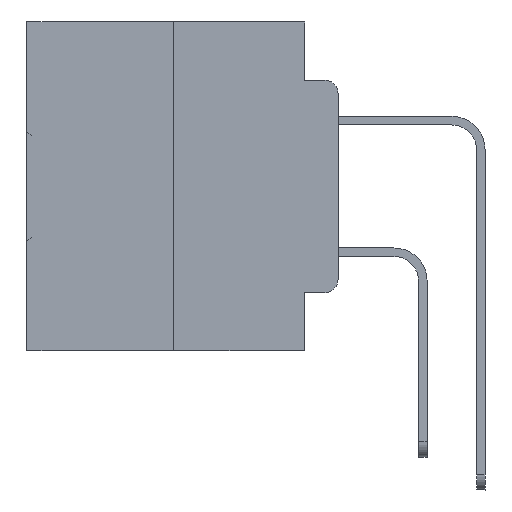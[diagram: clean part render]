
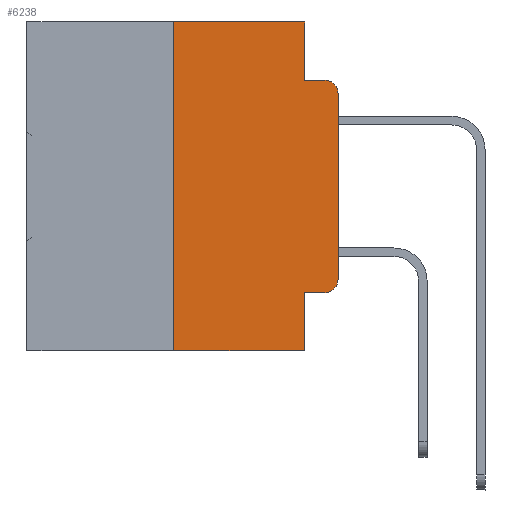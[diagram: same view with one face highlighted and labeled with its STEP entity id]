
A CAD part, left-side view. The second image highlights one B-rep face of the part: STEP entity #6238.
In plain terms, the highlighted planar face has unit normal (-1, 0, 0).
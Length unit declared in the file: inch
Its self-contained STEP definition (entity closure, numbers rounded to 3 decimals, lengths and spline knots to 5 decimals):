
#357 = VERTEX_POINT ( 'NONE', #23509 ) ;
#373 = PLANE ( 'NONE',  #26915 ) ;
#374 = VECTOR ( 'NONE', #2144, 39.37008 ) ;
#1751 = EDGE_CURVE ( 'NONE', #6356, #25258, #17116, .T. ) ;
#2144 = DIRECTION ( 'NONE',  ( 0., -1., 0. ) ) ;
#3812 = EDGE_CURVE ( 'NONE', #10874, #17082, #34216, .T. ) ;
#4017 = LINE ( 'NONE', #12427, #23844 ) ;
#5485 = VECTOR ( 'NONE', #8433, 39.37008 ) ;
#5541 = EDGE_CURVE ( 'NONE', #17421, #18664, #31424, .T. ) ;
#5869 = AXIS2_PLACEMENT_3D ( 'NONE', #33757, #22536, #11218 ) ;
#6238 = ADVANCED_FACE ( 'NONE', ( #25445 ), #373, .F. ) ;
#6356 = VERTEX_POINT ( 'NONE', #23574 ) ;
#7857 = CARTESIAN_POINT ( 'NONE',  ( 0., 0.051, 0. ) ) ;
#8274 = ORIENTED_EDGE ( 'NONE', *, *, #15475, .F. ) ;
#8433 = DIRECTION ( 'NONE',  ( 0., 0., -1. ) ) ;
#9820 = LINE ( 'NONE', #27207, #374 ) ;
#9904 = ORIENTED_EDGE ( 'NONE', *, *, #33420, .T. ) ;
#10700 = EDGE_CURVE ( 'NONE', #25258, #10874, #32923, .T. ) ;
#10799 = CARTESIAN_POINT ( 'NONE',  ( 0., 0.02, -0.3915 ) ) ;
#10874 = VERTEX_POINT ( 'NONE', #21183 ) ;
#10908 = CARTESIAN_POINT ( 'NONE',  ( 0., 0.25, 0. ) ) ;
#11174 = CARTESIAN_POINT ( 'NONE',  ( 0., 0.051, 0. ) ) ;
#11218 = DIRECTION ( 'NONE',  ( 0., 0., -1. ) ) ;
#11346 = LINE ( 'NONE', #11174, #5485 ) ;
#12414 = DIRECTION ( 'NONE',  ( 0., 0., 1. ) ) ;
#12427 = CARTESIAN_POINT ( 'NONE',  ( 0., 0.051, -0.0885 ) ) ;
#12939 = ORIENTED_EDGE ( 'NONE', *, *, #10700, .T. ) ;
#13610 = VECTOR ( 'NONE', #15141, 39.37008 ) ;
#13625 = CARTESIAN_POINT ( 'NONE',  ( 0., 0.051, -0.0885 ) ) ;
#14332 = VECTOR ( 'NONE', #24516, 39.37008 ) ;
#14453 = CARTESIAN_POINT ( 'NONE',  ( 0., 0.051, -0.5 ) ) ;
#14631 = CIRCLE ( 'NONE', #5869, 0.02 ) ;
#14952 = CARTESIAN_POINT ( 'NONE',  ( 0., 0.25, 0. ) ) ;
#15141 = DIRECTION ( 'NONE',  ( 0., 0., 1. ) ) ;
#15180 = DIRECTION ( 'NONE',  ( 0., -1., 0. ) ) ;
#15475 = EDGE_CURVE ( 'NONE', #6356, #31458, #11346, .T. ) ;
#15930 = LINE ( 'NONE', #7857, #14332 ) ;
#16313 = VECTOR ( 'NONE', #18277, 39.37008 ) ;
#16811 = EDGE_CURVE ( 'NONE', #357, #23910, #15930, .T. ) ;
#16850 = CARTESIAN_POINT ( 'NONE',  ( 0., 0.473, 0. ) ) ;
#17082 = VERTEX_POINT ( 'NONE', #29043 ) ;
#17116 = LINE ( 'NONE', #20376, #21104 ) ;
#17131 = AXIS2_PLACEMENT_3D ( 'NONE', #10799, #22118, #27281 ) ;
#17207 = DIRECTION ( 'NONE',  ( 1., 0., 0. ) ) ;
#17421 = VERTEX_POINT ( 'NONE', #20039 ) ;
#18277 = DIRECTION ( 'NONE',  ( 0., -1., 0. ) ) ;
#18637 = LINE ( 'NONE', #32922, #16313 ) ;
#18664 = VERTEX_POINT ( 'NONE', #10908 ) ;
#19331 = ORIENTED_EDGE ( 'NONE', *, *, #27562, .T. ) ;
#20039 = CARTESIAN_POINT ( 'NONE',  ( 0., 0.25, -0.5 ) ) ;
#20275 = CARTESIAN_POINT ( 'NONE',  ( 0., 0., 0. ) ) ;
#20376 = CARTESIAN_POINT ( 'NONE',  ( 0., 0.051, -0.4115 ) ) ;
#21104 = VECTOR ( 'NONE', #34315, 39.37008 ) ;
#21183 = CARTESIAN_POINT ( 'NONE',  ( 0., 0., -0.3915 ) ) ;
#21526 = EDGE_CURVE ( 'NONE', #23910, #23451, #4017, .T. ) ;
#22118 = DIRECTION ( 'NONE',  ( -1., 0., 0. ) ) ;
#22536 = DIRECTION ( 'NONE',  ( -1., 0., 0. ) ) ;
#23204 = CARTESIAN_POINT ( 'NONE',  ( 0., 0.02, -0.0885 ) ) ;
#23451 = VERTEX_POINT ( 'NONE', #23204 ) ;
#23509 = CARTESIAN_POINT ( 'NONE',  ( 0., 0.051, 0. ) ) ;
#23574 = CARTESIAN_POINT ( 'NONE',  ( 0., 0.051, -0.4115 ) ) ;
#23744 = VECTOR ( 'NONE', #12414, 39.37008 ) ;
#23844 = VECTOR ( 'NONE', #15180, 39.37008 ) ;
#23910 = VERTEX_POINT ( 'NONE', #13625 ) ;
#24214 = ORIENTED_EDGE ( 'NONE', *, *, #21526, .F. ) ;
#24516 = DIRECTION ( 'NONE',  ( 0., 0., -1. ) ) ;
#25258 = VERTEX_POINT ( 'NONE', #26196 ) ;
#25445 = FACE_OUTER_BOUND ( 'NONE', #31814, .T. ) ;
#26196 = CARTESIAN_POINT ( 'NONE',  ( 0., 0.02, -0.4115 ) ) ;
#26915 = AXIS2_PLACEMENT_3D ( 'NONE', #16850, #17207, #33881 ) ;
#27207 = CARTESIAN_POINT ( 'NONE',  ( 0., 0.473, -0.5 ) ) ;
#27281 = DIRECTION ( 'NONE',  ( 0., 0., -1. ) ) ;
#27562 = EDGE_CURVE ( 'NONE', #17421, #31458, #9820, .T. ) ;
#27658 = ORIENTED_EDGE ( 'NONE', *, *, #30386, .F. ) ;
#28955 = ORIENTED_EDGE ( 'NONE', *, *, #16811, .F. ) ;
#29043 = CARTESIAN_POINT ( 'NONE',  ( 0., 0., -0.1085 ) ) ;
#30386 = EDGE_CURVE ( 'NONE', #18664, #357, #18637, .T. ) ;
#30824 = ORIENTED_EDGE ( 'NONE', *, *, #5541, .F. ) ;
#31424 = LINE ( 'NONE', #14952, #13610 ) ;
#31458 = VERTEX_POINT ( 'NONE', #14453 ) ;
#31678 = ORIENTED_EDGE ( 'NONE', *, *, #1751, .T. ) ;
#31814 = EDGE_LOOP ( 'NONE', ( #33496, #9904, #24214, #28955, #27658, #30824, #19331, #8274, #31678, #12939 ) ) ;
#32922 = CARTESIAN_POINT ( 'NONE',  ( 0., 0.473, 0. ) ) ;
#32923 = CIRCLE ( 'NONE', #17131, 0.02 ) ;
#33420 = EDGE_CURVE ( 'NONE', #17082, #23451, #14631, .T. ) ;
#33496 = ORIENTED_EDGE ( 'NONE', *, *, #3812, .T. ) ;
#33757 = CARTESIAN_POINT ( 'NONE',  ( 0., 0.02, -0.1085 ) ) ;
#33881 = DIRECTION ( 'NONE',  ( 0., 0., -1. ) ) ;
#34216 = LINE ( 'NONE', #20275, #23744 ) ;
#34315 = DIRECTION ( 'NONE',  ( 0., -1., 0. ) ) ;
